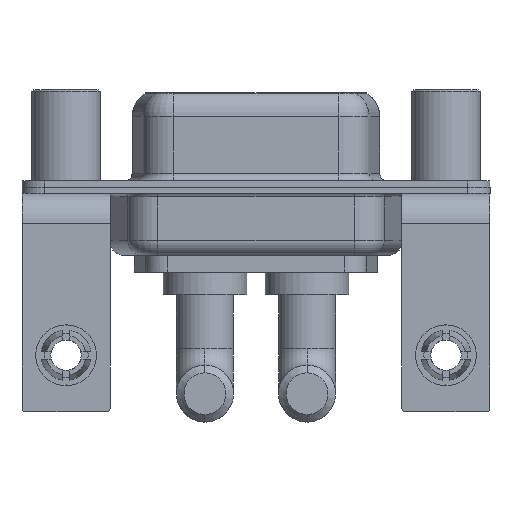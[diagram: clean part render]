
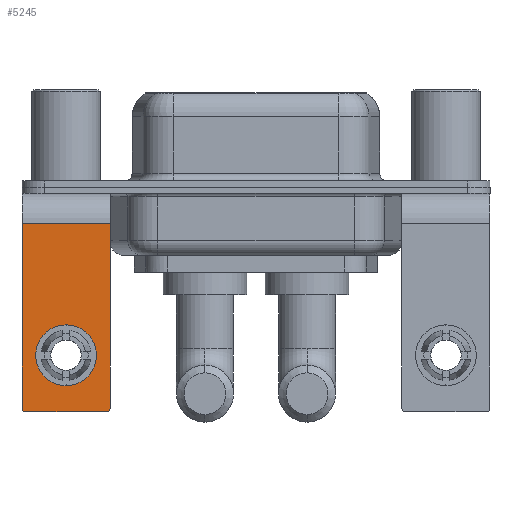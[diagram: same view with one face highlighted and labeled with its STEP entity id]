
A CAD part, front view. The second image highlights one B-rep face of the part: STEP entity #5245.
In plain terms, the highlighted planar face has unit normal (0, -1, 0).
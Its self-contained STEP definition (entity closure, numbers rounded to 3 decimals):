
#556 = CIRCLE ( 'NONE', #11972, 2. ) ;
#867 = EDGE_LOOP ( 'NONE', ( #11242, #10946 ) ) ;
#963 = AXIS2_PLACEMENT_3D ( 'NONE', #11097, #9912, #3871 ) ;
#1241 = DIRECTION ( 'NONE',  ( -1., 0., 0. ) ) ;
#1291 = EDGE_CURVE ( 'NONE', #3567, #13372, #3304, .T. ) ;
#1522 = EDGE_CURVE ( 'NONE', #7545, #5356, #4899, .T. ) ;
#1680 = EDGE_CURVE ( 'NONE', #3567, #3316, #7580, .T. ) ;
#2001 = DIRECTION ( 'NONE',  ( 0., 0., -1. ) ) ;
#2536 = FACE_OUTER_BOUND ( 'NONE', #14121, .T. ) ;
#2694 = VECTOR ( 'NONE', #5611, 1000. ) ;
#2844 = EDGE_CURVE ( 'NONE', #3392, #9198, #556, .T. ) ;
#2997 = VECTOR ( 'NONE', #2001, 1000. ) ;
#3304 = CIRCLE ( 'NONE', #12956, 0.25 ) ;
#3316 = VERTEX_POINT ( 'NONE', #7496 ) ;
#3344 = CARTESIAN_POINT ( 'NONE',  ( 2.9, -6.25, -2.4 ) ) ;
#3392 = VERTEX_POINT ( 'NONE', #13445 ) ;
#3560 = VECTOR ( 'NONE', #9104, 1000. ) ;
#3567 = VERTEX_POINT ( 'NONE', #4070 ) ;
#3866 = ORIENTED_EDGE ( 'NONE', *, *, #1522, .T. ) ;
#3871 = DIRECTION ( 'NONE',  ( 0., 0., 1. ) ) ;
#3927 = DIRECTION ( 'NONE',  ( 0., 0., 1. ) ) ;
#4070 = CARTESIAN_POINT ( 'NONE',  ( 2.65, -6.25, -14.8 ) ) ;
#4899 = LINE ( 'NONE', #9961, #8648 ) ;
#5245 = ADVANCED_FACE ( 'NONE', ( #13416, #2536 ), #7398, .F. ) ;
#5267 = ORIENTED_EDGE ( 'NONE', *, *, #1680, .F. ) ;
#5298 = CIRCLE ( 'NONE', #9854, 2. ) ;
#5356 = VERTEX_POINT ( 'NONE', #7628 ) ;
#5611 = DIRECTION ( 'NONE',  ( 0., 0., -1. ) ) ;
#5852 = ORIENTED_EDGE ( 'NONE', *, *, #11662, .F. ) ;
#5981 = LINE ( 'NONE', #3344, #2997 ) ;
#6097 = CARTESIAN_POINT ( 'NONE',  ( 2.9, -6.25, -2.4 ) ) ;
#6203 = DIRECTION ( 'NONE',  ( 0., 0., 1. ) ) ;
#6204 = DIRECTION ( 'NONE',  ( 0., 0., 1. ) ) ;
#6440 = CARTESIAN_POINT ( 'NONE',  ( 2.65, -6.25, -14.55 ) ) ;
#7398 = PLANE ( 'NONE',  #8204 ) ;
#7496 = CARTESIAN_POINT ( 'NONE',  ( -2.65, -6.25, -14.8 ) ) ;
#7545 = VERTEX_POINT ( 'NONE', #6097 ) ;
#7580 = LINE ( 'NONE', #7665, #3560 ) ;
#7628 = CARTESIAN_POINT ( 'NONE',  ( -2.9, -6.25, -2.4 ) ) ;
#7665 = CARTESIAN_POINT ( 'NONE',  ( 2.9, -6.25, -14.8 ) ) ;
#8201 = VERTEX_POINT ( 'NONE', #15266 ) ;
#8204 = AXIS2_PLACEMENT_3D ( 'NONE', #14538, #9849, #6203 ) ;
#8648 = VECTOR ( 'NONE', #1241, 1000. ) ;
#9104 = DIRECTION ( 'NONE',  ( -1., 0., 0. ) ) ;
#9198 = VERTEX_POINT ( 'NONE', #10518 ) ;
#9849 = DIRECTION ( 'NONE',  ( 0., 1., 0. ) ) ;
#9854 = AXIS2_PLACEMENT_3D ( 'NONE', #10579, #11764, #11836 ) ;
#9912 = DIRECTION ( 'NONE',  ( 0., -1., 0. ) ) ;
#9961 = CARTESIAN_POINT ( 'NONE',  ( 2.9, -6.25, -2.4 ) ) ;
#10518 = CARTESIAN_POINT ( 'NONE',  ( 0., -6.25, -9.07 ) ) ;
#10579 = CARTESIAN_POINT ( 'NONE',  ( 0., -6.25, -11.07 ) ) ;
#10946 = ORIENTED_EDGE ( 'NONE', *, *, #11591, .T. ) ;
#10985 = EDGE_CURVE ( 'NONE', #5356, #8201, #11468, .T. ) ;
#11097 = CARTESIAN_POINT ( 'NONE',  ( -2.65, -6.25, -14.55 ) ) ;
#11242 = ORIENTED_EDGE ( 'NONE', *, *, #2844, .T. ) ;
#11468 = LINE ( 'NONE', #15050, #2694 ) ;
#11591 = EDGE_CURVE ( 'NONE', #9198, #3392, #5298, .T. ) ;
#11662 = EDGE_CURVE ( 'NONE', #7545, #13372, #5981, .T. ) ;
#11764 = DIRECTION ( 'NONE',  ( 0., 1., 0. ) ) ;
#11836 = DIRECTION ( 'NONE',  ( 0., 0., 1. ) ) ;
#11972 = AXIS2_PLACEMENT_3D ( 'NONE', #13769, #14809, #3927 ) ;
#12295 = DIRECTION ( 'NONE',  ( 0., -1., 0. ) ) ;
#12443 = CARTESIAN_POINT ( 'NONE',  ( 2.9, -6.25, -14.55 ) ) ;
#12956 = AXIS2_PLACEMENT_3D ( 'NONE', #6440, #12295, #6204 ) ;
#13372 = VERTEX_POINT ( 'NONE', #12443 ) ;
#13416 = FACE_BOUND ( 'NONE', #867, .T. ) ;
#13445 = CARTESIAN_POINT ( 'NONE',  ( 0., -6.25, -13.07 ) ) ;
#13681 = ORIENTED_EDGE ( 'NONE', *, *, #14009, .T. ) ;
#13769 = CARTESIAN_POINT ( 'NONE',  ( 0., -6.25, -11.07 ) ) ;
#14009 = EDGE_CURVE ( 'NONE', #8201, #3316, #15674, .T. ) ;
#14121 = EDGE_LOOP ( 'NONE', ( #14521, #13681, #5267, #15080, #5852, #3866 ) ) ;
#14521 = ORIENTED_EDGE ( 'NONE', *, *, #10985, .T. ) ;
#14538 = CARTESIAN_POINT ( 'NONE',  ( 2.9, -6.25, -2.4 ) ) ;
#14809 = DIRECTION ( 'NONE',  ( 0., 1., 0. ) ) ;
#15050 = CARTESIAN_POINT ( 'NONE',  ( -2.9, -6.25, -2.4 ) ) ;
#15080 = ORIENTED_EDGE ( 'NONE', *, *, #1291, .T. ) ;
#15266 = CARTESIAN_POINT ( 'NONE',  ( -2.9, -6.25, -14.55 ) ) ;
#15674 = CIRCLE ( 'NONE', #963, 0.25 ) ;
